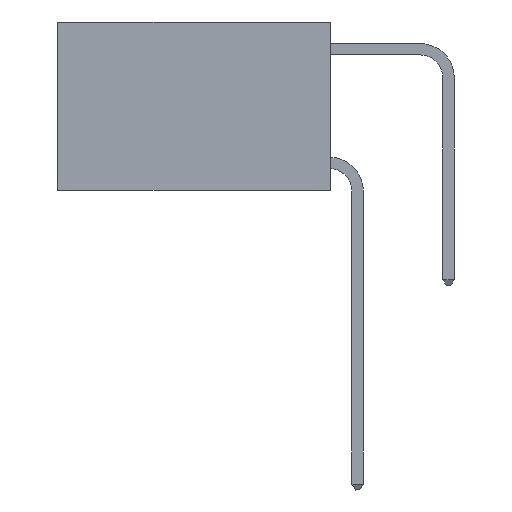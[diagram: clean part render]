
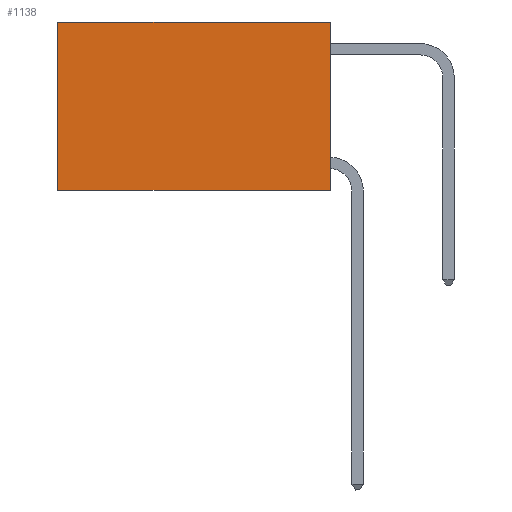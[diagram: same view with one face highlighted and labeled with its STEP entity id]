
A CAD part, left-side view. The second image highlights one B-rep face of the part: STEP entity #1138.
In plain terms, the highlighted planar face has unit normal (-1, 0, 0).
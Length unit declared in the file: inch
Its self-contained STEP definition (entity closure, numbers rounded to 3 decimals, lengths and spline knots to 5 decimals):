
#125 = VECTOR ( 'NONE', #3867, 39.37008 ) ;
#286 = EDGE_CURVE ( 'NONE', #10371, #15618, #7665, .T. ) ;
#529 = DIRECTION ( 'NONE',  ( 1., 0., 0. ) ) ;
#1138 = ADVANCED_FACE ( 'NONE', ( #14284 ), #7519, .F. ) ;
#1766 = VECTOR ( 'NONE', #8293, 39.37008 ) ;
#2157 = ORIENTED_EDGE ( 'NONE', *, *, #286, .F. ) ;
#2501 = DIRECTION ( 'NONE',  ( 0., 0., -1. ) ) ;
#3102 = LINE ( 'NONE', #9995, #1766 ) ;
#3867 = DIRECTION ( 'NONE',  ( 0., 0., -1. ) ) ;
#4074 = CARTESIAN_POINT ( 'NONE',  ( 0.2625, 0.6, 0. ) ) ;
#4437 = ORIENTED_EDGE ( 'NONE', *, *, #15260, .T. ) ;
#5148 = ORIENTED_EDGE ( 'NONE', *, *, #16868, .T. ) ;
#5903 = VERTEX_POINT ( 'NONE', #6904 ) ;
#5934 = DIRECTION ( 'NONE',  ( 0., 0., -1. ) ) ;
#6904 = CARTESIAN_POINT ( 'NONE',  ( 0.2625, 0.6, 0. ) ) ;
#7165 = CARTESIAN_POINT ( 'NONE',  ( 0.2625, 0., 0. ) ) ;
#7519 = PLANE ( 'NONE',  #20532 ) ;
#7665 = LINE ( 'NONE', #14546, #8246 ) ;
#7716 = CARTESIAN_POINT ( 'NONE',  ( 0.2625, 0., 0. ) ) ;
#8246 = VECTOR ( 'NONE', #16112, 39.37008 ) ;
#8293 = DIRECTION ( 'NONE',  ( 0., 1., 0. ) ) ;
#9094 = CARTESIAN_POINT ( 'NONE',  ( 0.2625, 0., 0. ) ) ;
#9995 = CARTESIAN_POINT ( 'NONE',  ( 0.2625, 0., 0. ) ) ;
#10371 = VERTEX_POINT ( 'NONE', #13963 ) ;
#10674 = LINE ( 'NONE', #7165, #125 ) ;
#10738 = CARTESIAN_POINT ( 'NONE',  ( 0.2625, 0.6, -0.37 ) ) ;
#10822 = EDGE_CURVE ( 'NONE', #17169, #10371, #10674, .T. ) ;
#13963 = CARTESIAN_POINT ( 'NONE',  ( 0.2625, 0., -0.37 ) ) ;
#14284 = FACE_OUTER_BOUND ( 'NONE', #18337, .T. ) ;
#14546 = CARTESIAN_POINT ( 'NONE',  ( 0.2625, 0., -0.37 ) ) ;
#15260 = EDGE_CURVE ( 'NONE', #5903, #15618, #17919, .T. ) ;
#15618 = VERTEX_POINT ( 'NONE', #10738 ) ;
#15789 = VECTOR ( 'NONE', #2501, 39.37008 ) ;
#16112 = DIRECTION ( 'NONE',  ( 0., 1., 0. ) ) ;
#16868 = EDGE_CURVE ( 'NONE', #17169, #5903, #3102, .T. ) ;
#17169 = VERTEX_POINT ( 'NONE', #7716 ) ;
#17919 = LINE ( 'NONE', #4074, #15789 ) ;
#18337 = EDGE_LOOP ( 'NONE', ( #4437, #2157, #19267, #5148 ) ) ;
#19267 = ORIENTED_EDGE ( 'NONE', *, *, #10822, .F. ) ;
#20532 = AXIS2_PLACEMENT_3D ( 'NONE', #9094, #529, #5934 ) ;
